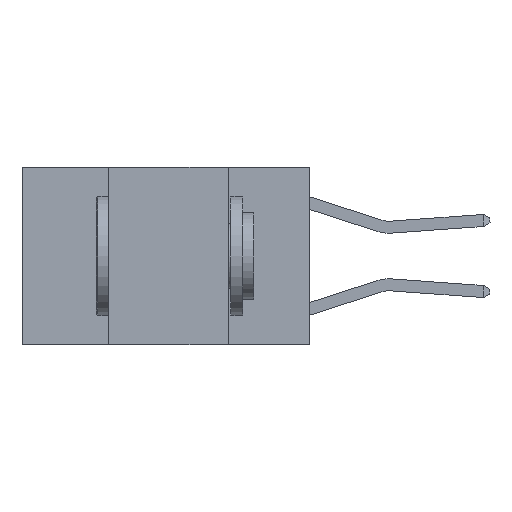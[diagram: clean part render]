
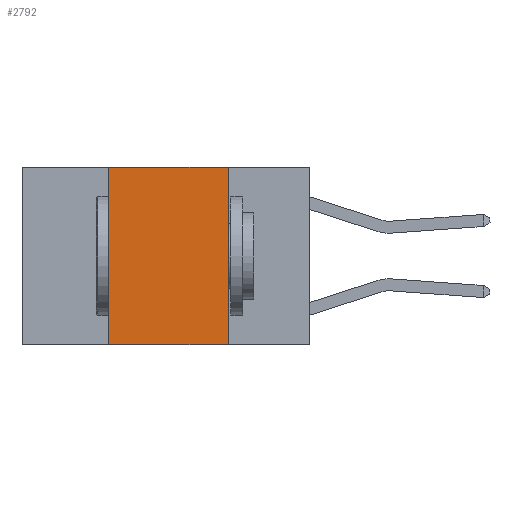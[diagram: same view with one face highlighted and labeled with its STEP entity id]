
A CAD part, left-side view. The second image highlights one B-rep face of the part: STEP entity #2792.
In plain terms, the highlighted planar face has unit normal (-1, 0, 0).
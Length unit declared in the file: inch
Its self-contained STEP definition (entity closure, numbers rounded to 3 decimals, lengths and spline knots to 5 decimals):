
#1039 = CARTESIAN_POINT ( 'NONE',  ( 0., 0.17, 0. ) ) ;
#1324 = CARTESIAN_POINT ( 'NONE',  ( 0., 0.17, -0.37 ) ) ;
#2161 = DIRECTION ( 'NONE',  ( 0., -1., 0. ) ) ;
#2382 = EDGE_CURVE ( 'NONE', #17751, #18525, #7057, .T. ) ;
#2433 = LINE ( 'NONE', #6650, #6369 ) ;
#2792 = ADVANCED_FACE ( 'NONE', ( #11377 ), #13777, .F. ) ;
#3237 = VERTEX_POINT ( 'NONE', #15110 ) ;
#3384 = EDGE_CURVE ( 'NONE', #7766, #3237, #2433, .T. ) ;
#4390 = VECTOR ( 'NONE', #15281, 39.37008 ) ;
#4866 = LINE ( 'NONE', #6509, #4390 ) ;
#5941 = LINE ( 'NONE', #12458, #10299 ) ;
#6369 = VECTOR ( 'NONE', #16906, 39.37008 ) ;
#6473 = CARTESIAN_POINT ( 'NONE',  ( 0., 0.6, 0. ) ) ;
#6509 = CARTESIAN_POINT ( 'NONE',  ( 0., 0.6, 0. ) ) ;
#6650 = CARTESIAN_POINT ( 'NONE',  ( 0., 0.42, 0. ) ) ;
#7057 = LINE ( 'NONE', #1039, #10931 ) ;
#7766 = VERTEX_POINT ( 'NONE', #15734 ) ;
#7942 = DIRECTION ( 'NONE',  ( 0., 0., -1. ) ) ;
#8312 = EDGE_CURVE ( 'NONE', #7766, #18525, #5941, .T. ) ;
#9033 = AXIS2_PLACEMENT_3D ( 'NONE', #6473, #16730, #7942 ) ;
#10116 = ORIENTED_EDGE ( 'NONE', *, *, #17413, .F. ) ;
#10299 = VECTOR ( 'NONE', #2161, 39.37008 ) ;
#10931 = VECTOR ( 'NONE', #12825, 39.37008 ) ;
#11377 = FACE_OUTER_BOUND ( 'NONE', #13715, .T. ) ;
#12129 = ORIENTED_EDGE ( 'NONE', *, *, #2382, .F. ) ;
#12458 = CARTESIAN_POINT ( 'NONE',  ( 0., 0.6, -0.37 ) ) ;
#12825 = DIRECTION ( 'NONE',  ( 0., 0., -1. ) ) ;
#12869 = ORIENTED_EDGE ( 'NONE', *, *, #3384, .F. ) ;
#13715 = EDGE_LOOP ( 'NONE', ( #12129, #10116, #12869, #14706 ) ) ;
#13777 = PLANE ( 'NONE',  #9033 ) ;
#14226 = CARTESIAN_POINT ( 'NONE',  ( 0., 0.17, 0. ) ) ;
#14706 = ORIENTED_EDGE ( 'NONE', *, *, #8312, .T. ) ;
#15110 = CARTESIAN_POINT ( 'NONE',  ( 0., 0.42, 0. ) ) ;
#15281 = DIRECTION ( 'NONE',  ( 0., -1., 0. ) ) ;
#15734 = CARTESIAN_POINT ( 'NONE',  ( 0., 0.42, -0.37 ) ) ;
#16730 = DIRECTION ( 'NONE',  ( 1., 0., 0. ) ) ;
#16906 = DIRECTION ( 'NONE',  ( 0., 0., 1. ) ) ;
#17413 = EDGE_CURVE ( 'NONE', #3237, #17751, #4866, .T. ) ;
#17751 = VERTEX_POINT ( 'NONE', #14226 ) ;
#18525 = VERTEX_POINT ( 'NONE', #1324 ) ;
